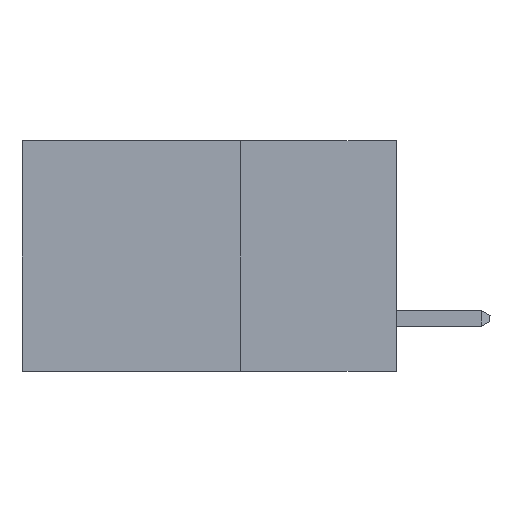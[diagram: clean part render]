
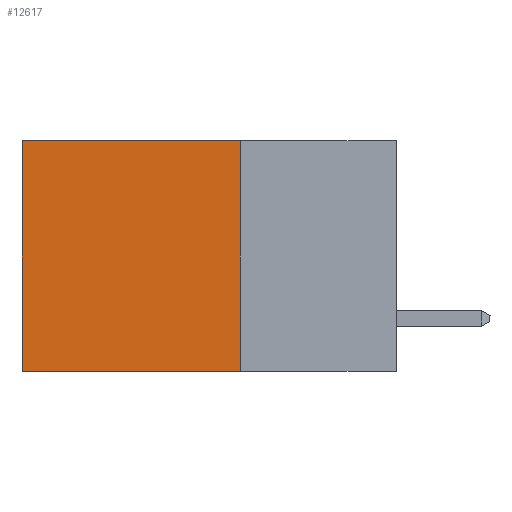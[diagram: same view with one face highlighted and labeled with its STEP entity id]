
A CAD part, left-side view. The second image highlights one B-rep face of the part: STEP entity #12617.
In plain terms, the highlighted planar face has unit normal (-1, 0, 0).
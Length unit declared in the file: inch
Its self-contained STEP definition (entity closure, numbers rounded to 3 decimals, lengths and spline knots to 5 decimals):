
#312 = DIRECTION ( 'NONE',  ( 0., 1., 0. ) ) ;
#369 = CARTESIAN_POINT ( 'NONE',  ( 0.2615, 0.25, -0.37 ) ) ;
#1481 = ORIENTED_EDGE ( 'NONE', *, *, #10068, .F. ) ;
#2961 = EDGE_LOOP ( 'NONE', ( #2985, #21128, #1481, #17348 ) ) ;
#2985 = ORIENTED_EDGE ( 'NONE', *, *, #17758, .T. ) ;
#3480 = DIRECTION ( 'NONE',  ( 0., 0., -1. ) ) ;
#3485 = DIRECTION ( 'NONE',  ( 1., 0., 0. ) ) ;
#3744 = PLANE ( 'NONE',  #19976 ) ;
#4129 = LINE ( 'NONE', #13754, #8059 ) ;
#4248 = CARTESIAN_POINT ( 'NONE',  ( 0.2615, 0.25, -0.37 ) ) ;
#5279 = CARTESIAN_POINT ( 'NONE',  ( 0.2615, 0.25, 0. ) ) ;
#7089 = CARTESIAN_POINT ( 'NONE',  ( 0.2615, 0.25, 0. ) ) ;
#8059 = VECTOR ( 'NONE', #17100, 39.37008 ) ;
#8446 = CARTESIAN_POINT ( 'NONE',  ( 0.2615, 0.6, -0.37 ) ) ;
#9296 = VERTEX_POINT ( 'NONE', #7089 ) ;
#9394 = CARTESIAN_POINT ( 'NONE',  ( 0.2615, 0.25, -0.37 ) ) ;
#9853 = LINE ( 'NONE', #369, #23767 ) ;
#9961 = EDGE_CURVE ( 'NONE', #11087, #14219, #9853, .T. ) ;
#10068 = EDGE_CURVE ( 'NONE', #9296, #11087, #4129, .T. ) ;
#11087 = VERTEX_POINT ( 'NONE', #9394 ) ;
#12617 = ADVANCED_FACE ( 'NONE', ( #14120 ), #3744, .F. ) ;
#12739 = LINE ( 'NONE', #8446, #17129 ) ;
#13048 = VERTEX_POINT ( 'NONE', #18171 ) ;
#13754 = CARTESIAN_POINT ( 'NONE',  ( 0.2615, 0.25, -0.37 ) ) ;
#14103 = DIRECTION ( 'NONE',  ( 0., 0., -1. ) ) ;
#14120 = FACE_OUTER_BOUND ( 'NONE', #2961, .T. ) ;
#14219 = VERTEX_POINT ( 'NONE', #20093 ) ;
#17100 = DIRECTION ( 'NONE',  ( 0., 0., -1. ) ) ;
#17129 = VECTOR ( 'NONE', #14103, 39.37008 ) ;
#17348 = ORIENTED_EDGE ( 'NONE', *, *, #18471, .T. ) ;
#17758 = EDGE_CURVE ( 'NONE', #13048, #14219, #12739, .T. ) ;
#18171 = CARTESIAN_POINT ( 'NONE',  ( 0.2615, 0.6, 0. ) ) ;
#18471 = EDGE_CURVE ( 'NONE', #9296, #13048, #23957, .T. ) ;
#19976 = AXIS2_PLACEMENT_3D ( 'NONE', #4248, #3485, #3480 ) ;
#20093 = CARTESIAN_POINT ( 'NONE',  ( 0.2615, 0.6, -0.37 ) ) ;
#20208 = DIRECTION ( 'NONE',  ( 0., 1., 0. ) ) ;
#21128 = ORIENTED_EDGE ( 'NONE', *, *, #9961, .F. ) ;
#23443 = VECTOR ( 'NONE', #20208, 39.37008 ) ;
#23767 = VECTOR ( 'NONE', #312, 39.37008 ) ;
#23957 = LINE ( 'NONE', #5279, #23443 ) ;
